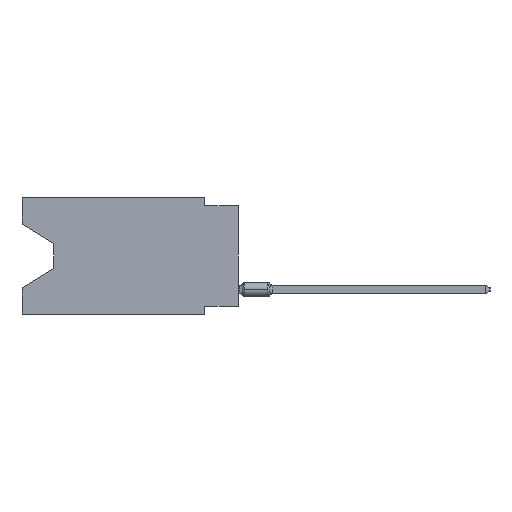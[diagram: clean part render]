
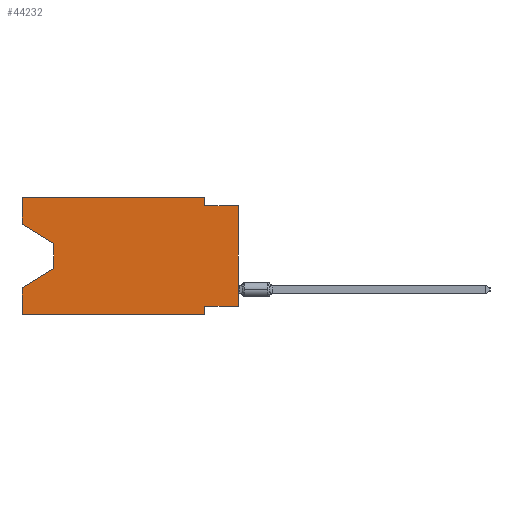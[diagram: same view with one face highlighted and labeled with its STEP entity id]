
A CAD part, left-side view. The second image highlights one B-rep face of the part: STEP entity #44232.
In plain terms, the highlighted planar face has unit normal (-1, 0, 0).
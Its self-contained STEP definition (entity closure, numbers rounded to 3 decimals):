
#525 = VECTOR ( 'NONE', #35086, 1000. ) ;
#3203 = CARTESIAN_POINT ( 'NONE',  ( 0., 16.383, 0. ) ) ;
#4183 = DIRECTION ( 'NONE',  ( 1., 0., 0. ) ) ;
#4610 = DIRECTION ( 'NONE',  ( 0., -1., 0. ) ) ;
#6045 = DIRECTION ( 'NONE',  ( 0., -1., 0. ) ) ;
#8327 = CARTESIAN_POINT ( 'NONE',  ( 0., 16.383, 0. ) ) ;
#8712 = VECTOR ( 'NONE', #4610, 1000. ) ;
#9271 = VERTEX_POINT ( 'NONE', #77582 ) ;
#13326 = CARTESIAN_POINT ( 'NONE',  ( 0., 0., -0.635 ) ) ;
#16460 = VECTOR ( 'NONE', #16622, 1000. ) ;
#16622 = DIRECTION ( 'NONE',  ( 0., 0., 1. ) ) ;
#17561 = CARTESIAN_POINT ( 'NONE',  ( 0., 0., 0. ) ) ;
#18290 = CARTESIAN_POINT ( 'NONE',  ( 0., 13.97, -5.385 ) ) ;
#19257 = CARTESIAN_POINT ( 'NONE',  ( 0., 2.54, -8.89 ) ) ;
#20182 = LINE ( 'NONE', #26828, #31078 ) ;
#20237 = DIRECTION ( 'NONE',  ( 0., 0., -1. ) ) ;
#21510 = CARTESIAN_POINT ( 'NONE',  ( 0., 0., -8.255 ) ) ;
#23934 = ORIENTED_EDGE ( 'NONE', *, *, #24228, .F. ) ;
#24228 = EDGE_CURVE ( 'NONE', #79584, #46545, #69900, .T. ) ;
#26037 = DIRECTION ( 'NONE',  ( 0., 0., -1. ) ) ;
#26828 = CARTESIAN_POINT ( 'NONE',  ( 0., 13.97, -5.385 ) ) ;
#26890 = PLANE ( 'NONE',  #86090 ) ;
#28165 = DIRECTION ( 'NONE',  ( 0., 1., 0. ) ) ;
#28538 = VECTOR ( 'NONE', #6045, 1000. ) ;
#29457 = EDGE_CURVE ( 'NONE', #31300, #79584, #50939, .T. ) ;
#31051 = DIRECTION ( 'NONE',  ( 0., 0., 1. ) ) ;
#31078 = VECTOR ( 'NONE', #55717, 1000. ) ;
#31300 = VERTEX_POINT ( 'NONE', #38535 ) ;
#31389 = ORIENTED_EDGE ( 'NONE', *, *, #44706, .F. ) ;
#31470 = VERTEX_POINT ( 'NONE', #76395 ) ;
#31697 = EDGE_CURVE ( 'NONE', #46545, #31470, #37476, .T. ) ;
#34064 = CARTESIAN_POINT ( 'NONE',  ( 0., 2.54, -8.89 ) ) ;
#34281 = ORIENTED_EDGE ( 'NONE', *, *, #86553, .T. ) ;
#35086 = DIRECTION ( 'NONE',  ( 0., -1., 0. ) ) ;
#35519 = VECTOR ( 'NONE', #74192, 1000. ) ;
#37379 = VECTOR ( 'NONE', #26037, 1000. ) ;
#37415 = VERTEX_POINT ( 'NONE', #13326 ) ;
#37476 = LINE ( 'NONE', #67770, #85668 ) ;
#38535 = CARTESIAN_POINT ( 'NONE',  ( 0., 16.383, -2.038 ) ) ;
#39431 = VERTEX_POINT ( 'NONE', #70192 ) ;
#40386 = ORIENTED_EDGE ( 'NONE', *, *, #65648, .T. ) ;
#40722 = CARTESIAN_POINT ( 'NONE',  ( 0., 2.54, -8.255 ) ) ;
#44232 = ADVANCED_FACE ( 'NONE', ( #69029 ), #26890, .F. ) ;
#44706 = EDGE_CURVE ( 'NONE', #54099, #73074, #50383, .T. ) ;
#46278 = LINE ( 'NONE', #3203, #35519 ) ;
#46545 = VERTEX_POINT ( 'NONE', #90200 ) ;
#47676 = ORIENTED_EDGE ( 'NONE', *, *, #29457, .F. ) ;
#47754 = VECTOR ( 'NONE', #58010, 1000. ) ;
#48831 = LINE ( 'NONE', #92844, #525 ) ;
#50361 = ORIENTED_EDGE ( 'NONE', *, *, #84758, .F. ) ;
#50383 = LINE ( 'NONE', #21510, #56024 ) ;
#50939 = LINE ( 'NONE', #8327, #59412 ) ;
#53167 = CARTESIAN_POINT ( 'NONE',  ( 0., 13.97, -3.505 ) ) ;
#53614 = CARTESIAN_POINT ( 'NONE',  ( 0., 16.383, -2.038 ) ) ;
#54099 = VERTEX_POINT ( 'NONE', #79266 ) ;
#55483 = ORIENTED_EDGE ( 'NONE', *, *, #31697, .F. ) ;
#55717 = DIRECTION ( 'NONE',  ( 0., 0.855, -0.519 ) ) ;
#56024 = VECTOR ( 'NONE', #28165, 1000. ) ;
#56748 = ORIENTED_EDGE ( 'NONE', *, *, #76492, .F. ) ;
#57839 = ORIENTED_EDGE ( 'NONE', *, *, #75265, .T. ) ;
#58010 = DIRECTION ( 'NONE',  ( 0., 0., -1. ) ) ;
#59412 = VECTOR ( 'NONE', #31051, 1000. ) ;
#60781 = CARTESIAN_POINT ( 'NONE',  ( 0., 16.383, 0. ) ) ;
#64636 = VERTEX_POINT ( 'NONE', #53167 ) ;
#65582 = CARTESIAN_POINT ( 'NONE',  ( 0., 13.97, -3.505 ) ) ;
#65645 = LINE ( 'NONE', #93586, #28538 ) ;
#65648 = EDGE_CURVE ( 'NONE', #54099, #37415, #66333, .T. ) ;
#66333 = LINE ( 'NONE', #17561, #16460 ) ;
#67770 = CARTESIAN_POINT ( 'NONE',  ( 0., 2.54, 0. ) ) ;
#69029 = FACE_OUTER_BOUND ( 'NONE', #86316, .T. ) ;
#69900 = LINE ( 'NONE', #91695, #8712 ) ;
#70192 = CARTESIAN_POINT ( 'NONE',  ( 0., 16.383, -8.89 ) ) ;
#73074 = VERTEX_POINT ( 'NONE', #40722 ) ;
#73335 = VECTOR ( 'NONE', #84352, 1000. ) ;
#74192 = DIRECTION ( 'NONE',  ( 0., 0., 1. ) ) ;
#75265 = EDGE_CURVE ( 'NONE', #64636, #81942, #88296, .T. ) ;
#76395 = CARTESIAN_POINT ( 'NONE',  ( 0., 2.54, -0.635 ) ) ;
#76492 = EDGE_CURVE ( 'NONE', #73074, #86490, #90893, .T. ) ;
#77283 = ORIENTED_EDGE ( 'NONE', *, *, #88956, .F. ) ;
#77582 = CARTESIAN_POINT ( 'NONE',  ( 0., 16.383, -6.852 ) ) ;
#77804 = EDGE_CURVE ( 'NONE', #39431, #86490, #65645, .T. ) ;
#79266 = CARTESIAN_POINT ( 'NONE',  ( 0., 0., -8.255 ) ) ;
#79584 = VERTEX_POINT ( 'NONE', #60781 ) ;
#80495 = ORIENTED_EDGE ( 'NONE', *, *, #77804, .T. ) ;
#81942 = VERTEX_POINT ( 'NONE', #18290 ) ;
#84352 = DIRECTION ( 'NONE',  ( 0., -0.855, -0.519 ) ) ;
#84758 = EDGE_CURVE ( 'NONE', #39431, #9271, #46278, .T. ) ;
#85098 = CARTESIAN_POINT ( 'NONE',  ( 0., 16.383, 0. ) ) ;
#85668 = VECTOR ( 'NONE', #88608, 1000. ) ;
#86090 = AXIS2_PLACEMENT_3D ( 'NONE', #85098, #4183, #20237 ) ;
#86316 = EDGE_LOOP ( 'NONE', ( #87375, #57839, #34281, #50361, #80495, #56748, #31389, #40386, #77283, #55483, #23934, #47676 ) ) ;
#86490 = VERTEX_POINT ( 'NONE', #19257 ) ;
#86553 = EDGE_CURVE ( 'NONE', #81942, #9271, #20182, .T. ) ;
#87375 = ORIENTED_EDGE ( 'NONE', *, *, #92663, .T. ) ;
#88296 = LINE ( 'NONE', #65582, #47754 ) ;
#88608 = DIRECTION ( 'NONE',  ( 0., 0., -1. ) ) ;
#88956 = EDGE_CURVE ( 'NONE', #31470, #37415, #48831, .T. ) ;
#90053 = LINE ( 'NONE', #53614, #73335 ) ;
#90200 = CARTESIAN_POINT ( 'NONE',  ( 0., 2.54, 0. ) ) ;
#90893 = LINE ( 'NONE', #34064, #37379 ) ;
#91695 = CARTESIAN_POINT ( 'NONE',  ( 0., 16.383, 0. ) ) ;
#92663 = EDGE_CURVE ( 'NONE', #31300, #64636, #90053, .T. ) ;
#92844 = CARTESIAN_POINT ( 'NONE',  ( 0., 0., -0.635 ) ) ;
#93586 = CARTESIAN_POINT ( 'NONE',  ( 0., 16.383, -8.89 ) ) ;
